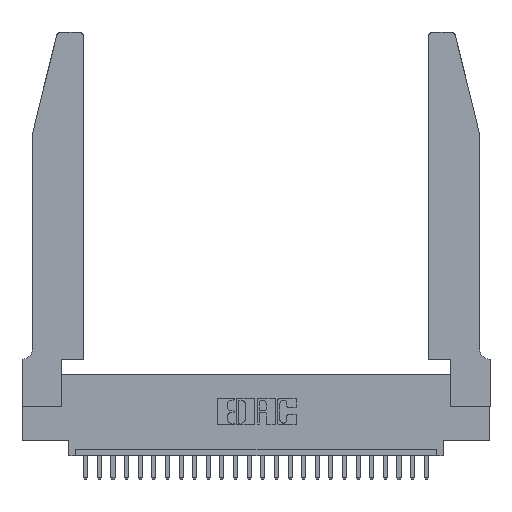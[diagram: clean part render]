
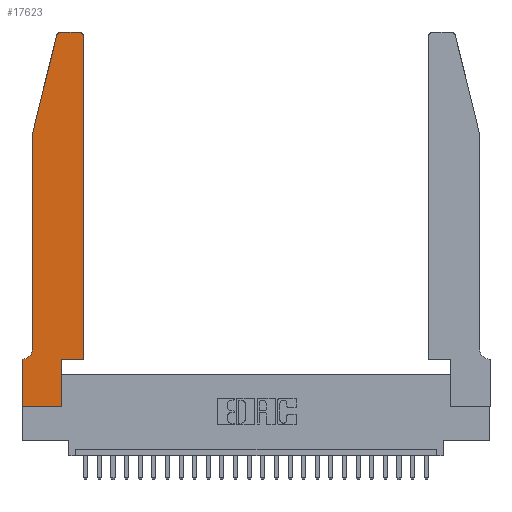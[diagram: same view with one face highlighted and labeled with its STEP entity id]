
A CAD part, top view. The second image highlights one B-rep face of the part: STEP entity #17623.
In plain terms, the highlighted planar face has unit normal (0, 0, 1).
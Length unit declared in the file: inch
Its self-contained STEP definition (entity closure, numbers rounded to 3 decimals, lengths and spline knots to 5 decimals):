
#347 = ORIENTED_EDGE ( 'NONE', *, *, #5920, .T. ) ;
#774 = CARTESIAN_POINT ( 'NONE',  ( 0.2605, 2.75, 0.37 ) ) ;
#1092 = DIRECTION ( 'NONE',  ( 0., 0., -1. ) ) ;
#1274 = ORIENTED_EDGE ( 'NONE', *, *, #13199, .T. ) ;
#1635 = ORIENTED_EDGE ( 'NONE', *, *, #23105, .T. ) ;
#1677 = CARTESIAN_POINT ( 'NONE',  ( 0., 0.35, 0.37 ) ) ;
#2115 = DIRECTION ( 'NONE',  ( 1., 0., 0. ) ) ;
#2194 = CARTESIAN_POINT ( 'NONE',  ( 0., 0., 0.37 ) ) ;
#2351 = LINE ( 'NONE', #16033, #23631 ) ;
#3025 = DIRECTION ( 'NONE',  ( -1., 0., 0. ) ) ;
#3543 = LINE ( 'NONE', #774, #6178 ) ;
#3645 = CARTESIAN_POINT ( 'NONE',  ( 0.284, 2.72, 0.37 ) ) ;
#3803 = EDGE_CURVE ( 'NONE', #16585, #4339, #20875, .T. ) ;
#3843 = DIRECTION ( 'NONE',  ( 1., 0., 0. ) ) ;
#3947 = ORIENTED_EDGE ( 'NONE', *, *, #17972, .T. ) ;
#4339 = VERTEX_POINT ( 'NONE', #8203 ) ;
#4480 = VECTOR ( 'NONE', #20999, 39.37008 ) ;
#4507 = AXIS2_PLACEMENT_3D ( 'NONE', #17388, #1092, #3025 ) ;
#5060 = CARTESIAN_POINT ( 'NONE',  ( 0.2865, 0.35, 0.37 ) ) ;
#5212 = ORIENTED_EDGE ( 'NONE', *, *, #17697, .T. ) ;
#5793 = DIRECTION ( 'NONE',  ( 1., 0., 0. ) ) ;
#5896 = VECTOR ( 'NONE', #19896, 39.37008 ) ;
#5920 = EDGE_CURVE ( 'NONE', #14141, #15691, #16110, .T. ) ;
#6178 = VECTOR ( 'NONE', #8912, 39.37008 ) ;
#6872 = LINE ( 'NONE', #21605, #5896 ) ;
#7173 = CARTESIAN_POINT ( 'NONE',  ( 0., 0., 0.37 ) ) ;
#7664 = VECTOR ( 'NONE', #2115, 39.37008 ) ;
#7709 = VECTOR ( 'NONE', #12379, 39.37008 ) ;
#8020 = EDGE_CURVE ( 'NONE', #26525, #8866, #13117, .T. ) ;
#8198 = AXIS2_PLACEMENT_3D ( 'NONE', #3645, #18354, #26687 ) ;
#8203 = CARTESIAN_POINT ( 'NONE',  ( 0.4505, 2.72, 0.37 ) ) ;
#8286 = CARTESIAN_POINT ( 'NONE',  ( 0.2865, 0., 0.37 ) ) ;
#8861 = VERTEX_POINT ( 'NONE', #11880 ) ;
#8866 = VERTEX_POINT ( 'NONE', #8286 ) ;
#8912 = DIRECTION ( 'NONE',  ( -1., 0., 0. ) ) ;
#9638 = CARTESIAN_POINT ( 'NONE',  ( 0.4505, 0.35, 0.37 ) ) ;
#9920 = DIRECTION ( 'NONE',  ( 0., -1., 0. ) ) ;
#10108 = CARTESIAN_POINT ( 'NONE',  ( 0.0055, 0.35, 0.37 ) ) ;
#10350 = VERTEX_POINT ( 'NONE', #26738 ) ;
#10368 = VECTOR ( 'NONE', #17616, 39.37008 ) ;
#11468 = FACE_OUTER_BOUND ( 'NONE', #19337, .T. ) ;
#11627 = ORIENTED_EDGE ( 'NONE', *, *, #12647, .T. ) ;
#11685 = LINE ( 'NONE', #15446, #10368 ) ;
#11880 = CARTESIAN_POINT ( 'NONE',  ( 0.0755, 2., 0.37 ) ) ;
#12128 = VERTEX_POINT ( 'NONE', #15204 ) ;
#12159 = DIRECTION ( 'NONE',  ( 0., 1., 0. ) ) ;
#12379 = DIRECTION ( 'NONE',  ( 0., -1., 0. ) ) ;
#12647 = EDGE_CURVE ( 'NONE', #15691, #8861, #6872, .T. ) ;
#12948 = ORIENTED_EDGE ( 'NONE', *, *, #3803, .T. ) ;
#12975 = ORIENTED_EDGE ( 'NONE', *, *, #19775, .T. ) ;
#13117 = LINE ( 'NONE', #24980, #7664 ) ;
#13199 = EDGE_CURVE ( 'NONE', #18860, #16297, #11685, .T. ) ;
#13716 = VECTOR ( 'NONE', #12159, 39.37008 ) ;
#13820 = LINE ( 'NONE', #2194, #7709 ) ;
#14054 = CIRCLE ( 'NONE', #24783, 0.03 ) ;
#14141 = VERTEX_POINT ( 'NONE', #18847 ) ;
#14381 = ORIENTED_EDGE ( 'NONE', *, *, #22443, .T. ) ;
#15204 = CARTESIAN_POINT ( 'NONE',  ( 0.0755, 0.42, 0.37 ) ) ;
#15446 = CARTESIAN_POINT ( 'NONE',  ( 0.0755, 0.35, 0.37 ) ) ;
#15691 = VERTEX_POINT ( 'NONE', #23575 ) ;
#15701 = DIRECTION ( 'NONE',  ( 1., 0., 0. ) ) ;
#16033 = CARTESIAN_POINT ( 'NONE',  ( 0.4505, 0.35, 0.37 ) ) ;
#16110 = CIRCLE ( 'NONE', #8198, 0.03 ) ;
#16297 = VERTEX_POINT ( 'NONE', #1677 ) ;
#16585 = VERTEX_POINT ( 'NONE', #9638 ) ;
#16952 = AXIS2_PLACEMENT_3D ( 'NONE', #22285, #18372, #3843 ) ;
#17388 = CARTESIAN_POINT ( 'NONE',  ( 0.0055, 0.42, 0.37 ) ) ;
#17616 = DIRECTION ( 'NONE',  ( -1., 0., 0. ) ) ;
#17623 = ADVANCED_FACE ( 'NONE', ( #11468 ), #18198, .T. ) ;
#17697 = EDGE_CURVE ( 'NONE', #20574, #16585, #2351, .T. ) ;
#17916 = CARTESIAN_POINT ( 'NONE',  ( 0.2865, 0.35, 0.37 ) ) ;
#17972 = EDGE_CURVE ( 'NONE', #12128, #18860, #25018, .T. ) ;
#18198 = PLANE ( 'NONE',  #16952 ) ;
#18354 = DIRECTION ( 'NONE',  ( 0., 0., 1. ) ) ;
#18372 = DIRECTION ( 'NONE',  ( 0., 0., 1. ) ) ;
#18847 = CARTESIAN_POINT ( 'NONE',  ( 0.284, 2.75, 0.37 ) ) ;
#18860 = VERTEX_POINT ( 'NONE', #10108 ) ;
#19149 = LINE ( 'NONE', #17916, #13716 ) ;
#19337 = EDGE_LOOP ( 'NONE', ( #12975, #347, #11627, #23658, #3947, #1274, #22811, #25495, #1635, #5212, #12948, #14381 ) ) ;
#19775 = EDGE_CURVE ( 'NONE', #10350, #14141, #3543, .T. ) ;
#19885 = VECTOR ( 'NONE', #9920, 39.37008 ) ;
#19896 = DIRECTION ( 'NONE',  ( -0.239, -0.971, 0. ) ) ;
#20079 = DIRECTION ( 'NONE',  ( 0., 0., 1. ) ) ;
#20574 = VERTEX_POINT ( 'NONE', #5060 ) ;
#20875 = LINE ( 'NONE', #25005, #4480 ) ;
#20999 = DIRECTION ( 'NONE',  ( 0., 1., 0. ) ) ;
#21605 = CARTESIAN_POINT ( 'NONE',  ( 0.0755, 2., 0.37 ) ) ;
#22285 = CARTESIAN_POINT ( 'NONE',  ( 0., 0.35, 0.37 ) ) ;
#22433 = CARTESIAN_POINT ( 'NONE',  ( 0.0755, 2., 0.37 ) ) ;
#22443 = EDGE_CURVE ( 'NONE', #4339, #10350, #14054, .T. ) ;
#22811 = ORIENTED_EDGE ( 'NONE', *, *, #24847, .T. ) ;
#23105 = EDGE_CURVE ( 'NONE', #8866, #20574, #19149, .T. ) ;
#23575 = CARTESIAN_POINT ( 'NONE',  ( 0.25487, 2.72718, 0.37 ) ) ;
#23631 = VECTOR ( 'NONE', #5793, 39.37008 ) ;
#23658 = ORIENTED_EDGE ( 'NONE', *, *, #25347, .T. ) ;
#24783 = AXIS2_PLACEMENT_3D ( 'NONE', #26092, #20079, #15701 ) ;
#24847 = EDGE_CURVE ( 'NONE', #16297, #26525, #13820, .T. ) ;
#24980 = CARTESIAN_POINT ( 'NONE',  ( 0., 0., 0.37 ) ) ;
#25005 = CARTESIAN_POINT ( 'NONE',  ( 0.4505, 0.35, 0.37 ) ) ;
#25018 = CIRCLE ( 'NONE', #4507, 0.07 ) ;
#25312 = LINE ( 'NONE', #22433, #19885 ) ;
#25347 = EDGE_CURVE ( 'NONE', #8861, #12128, #25312, .T. ) ;
#25495 = ORIENTED_EDGE ( 'NONE', *, *, #8020, .T. ) ;
#26092 = CARTESIAN_POINT ( 'NONE',  ( 0.4205, 2.72, 0.37 ) ) ;
#26525 = VERTEX_POINT ( 'NONE', #7173 ) ;
#26687 = DIRECTION ( 'NONE',  ( 1., 0., 0. ) ) ;
#26738 = CARTESIAN_POINT ( 'NONE',  ( 0.4205, 2.75, 0.37 ) ) ;
